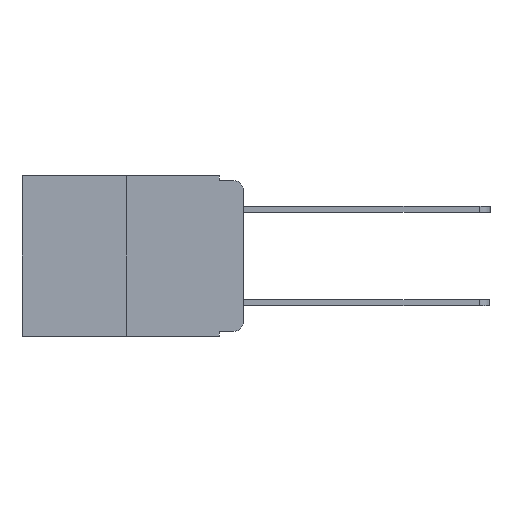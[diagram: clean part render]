
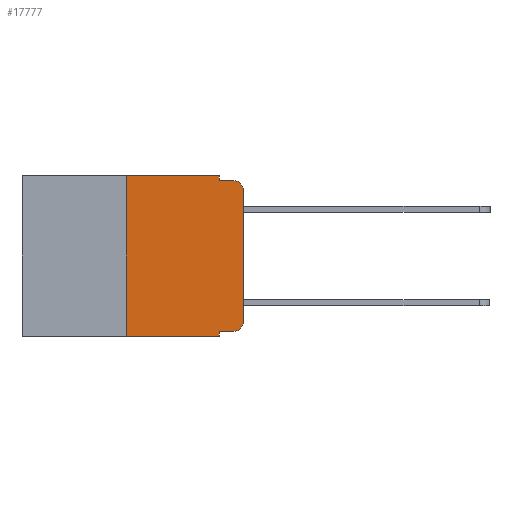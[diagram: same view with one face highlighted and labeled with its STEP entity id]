
A CAD part, left-side view. The second image highlights one B-rep face of the part: STEP entity #17777.
In plain terms, the highlighted planar face has unit normal (-1, 0, 0).
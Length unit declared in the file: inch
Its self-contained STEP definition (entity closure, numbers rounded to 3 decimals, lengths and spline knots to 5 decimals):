
#279 = VECTOR ( 'NONE', #8075, 39.37008 ) ;
#639 = ORIENTED_EDGE ( 'NONE', *, *, #17672, .T. ) ;
#662 = VERTEX_POINT ( 'NONE', #15641 ) ;
#718 = DIRECTION ( 'NONE',  ( 0., -1., 0. ) ) ;
#961 = AXIS2_PLACEMENT_3D ( 'NONE', #13818, #5654, #15170 ) ;
#1126 = AXIS2_PLACEMENT_3D ( 'NONE', #16324, #8238, #17665 ) ;
#1350 = ORIENTED_EDGE ( 'NONE', *, *, #10837, .F. ) ;
#1382 = PLANE ( 'NONE',  #961 ) ;
#1515 = CARTESIAN_POINT ( 'NONE',  ( 0., 0., -0.313 ) ) ;
#1614 = FACE_OUTER_BOUND ( 'NONE', #2027, .T. ) ;
#1800 = ORIENTED_EDGE ( 'NONE', *, *, #10014, .T. ) ;
#2027 = EDGE_LOOP ( 'NONE', ( #1800, #17594, #4031, #15746, #5764, #1350, #6407, #3618, #639, #6210 ) ) ;
#2047 = CARTESIAN_POINT ( 'NONE',  ( 0., 0.051, -0.343 ) ) ;
#2049 = DIRECTION ( 'NONE',  ( -1., 0., 0. ) ) ;
#2237 = VECTOR ( 'NONE', #15881, 39.37008 ) ;
#2392 = DIRECTION ( 'NONE',  ( 0., -1., 0. ) ) ;
#2447 = CIRCLE ( 'NONE', #1126, 0.02 ) ;
#2572 = VERTEX_POINT ( 'NONE', #16984 ) ;
#2578 = VECTOR ( 'NONE', #5127, 39.37008 ) ;
#2597 = CARTESIAN_POINT ( 'NONE',  ( 0., 0.051, -0.333 ) ) ;
#2837 = VERTEX_POINT ( 'NONE', #9090 ) ;
#3618 = ORIENTED_EDGE ( 'NONE', *, *, #13225, .F. ) ;
#3702 = CARTESIAN_POINT ( 'NONE',  ( 0., 0.051, -0.01 ) ) ;
#3815 = CARTESIAN_POINT ( 'NONE',  ( 0., 0., -0.03 ) ) ;
#3895 = VERTEX_POINT ( 'NONE', #6278 ) ;
#4012 = DIRECTION ( 'NONE',  ( 0., -1., 0. ) ) ;
#4031 = ORIENTED_EDGE ( 'NONE', *, *, #7508, .F. ) ;
#4441 = CARTESIAN_POINT ( 'NONE',  ( 0., 0.051, 0. ) ) ;
#4512 = CARTESIAN_POINT ( 'NONE',  ( 0., 0.25, 0. ) ) ;
#4763 = VECTOR ( 'NONE', #15292, 39.37008 ) ;
#5018 = CARTESIAN_POINT ( 'NONE',  ( 0., 0.051, 0. ) ) ;
#5127 = DIRECTION ( 'NONE',  ( 0., -1., 0. ) ) ;
#5654 = DIRECTION ( 'NONE',  ( 1., 0., 0. ) ) ;
#5764 = ORIENTED_EDGE ( 'NONE', *, *, #13348, .F. ) ;
#5766 = LINE ( 'NONE', #4441, #8536 ) ;
#6210 = ORIENTED_EDGE ( 'NONE', *, *, #8307, .T. ) ;
#6259 = CIRCLE ( 'NONE', #12583, 0.02 ) ;
#6276 = LINE ( 'NONE', #13308, #2578 ) ;
#6278 = CARTESIAN_POINT ( 'NONE',  ( 0., 0.051, 0. ) ) ;
#6372 = LINE ( 'NONE', #5018, #2237 ) ;
#6392 = VECTOR ( 'NONE', #718, 39.37008 ) ;
#6407 = ORIENTED_EDGE ( 'NONE', *, *, #10538, .T. ) ;
#6731 = CARTESIAN_POINT ( 'NONE',  ( 0., 0., 0. ) ) ;
#7066 = VECTOR ( 'NONE', #4012, 39.37008 ) ;
#7508 = EDGE_CURVE ( 'NONE', #16400, #7605, #14688, .T. ) ;
#7605 = VERTEX_POINT ( 'NONE', #13563 ) ;
#7802 = LINE ( 'NONE', #6731, #279 ) ;
#7900 = CARTESIAN_POINT ( 'NONE',  ( 0., 0.051, -0.01 ) ) ;
#8075 = DIRECTION ( 'NONE',  ( 0., 0., 1. ) ) ;
#8078 = EDGE_CURVE ( 'NONE', #3895, #16400, #6372, .T. ) ;
#8238 = DIRECTION ( 'NONE',  ( -1., 0., 0. ) ) ;
#8307 = EDGE_CURVE ( 'NONE', #2572, #13183, #2447, .T. ) ;
#8391 = LINE ( 'NONE', #13955, #4763 ) ;
#8536 = VECTOR ( 'NONE', #15351, 39.37008 ) ;
#9090 = CARTESIAN_POINT ( 'NONE',  ( 0., 0.051, -0.333 ) ) ;
#9122 = CARTESIAN_POINT ( 'NONE',  ( 0., 0.473, 0. ) ) ;
#10014 = EDGE_CURVE ( 'NONE', #13183, #12296, #7802, .T. ) ;
#10041 = LINE ( 'NONE', #9122, #6392 ) ;
#10344 = CARTESIAN_POINT ( 'NONE',  ( 0., 0.02, -0.03 ) ) ;
#10538 = EDGE_CURVE ( 'NONE', #662, #12791, #6276, .T. ) ;
#10837 = EDGE_CURVE ( 'NONE', #662, #10880, #8391, .T. ) ;
#10880 = VERTEX_POINT ( 'NONE', #4512 ) ;
#11088 = VECTOR ( 'NONE', #2392, 39.37008 ) ;
#11169 = LINE ( 'NONE', #2597, #7066 ) ;
#11727 = DIRECTION ( 'NONE',  ( 0., 0., -1. ) ) ;
#12296 = VERTEX_POINT ( 'NONE', #3815 ) ;
#12583 = AXIS2_PLACEMENT_3D ( 'NONE', #10344, #2049, #11727 ) ;
#12791 = VERTEX_POINT ( 'NONE', #2047 ) ;
#13183 = VERTEX_POINT ( 'NONE', #1515 ) ;
#13225 = EDGE_CURVE ( 'NONE', #2837, #12791, #5766, .T. ) ;
#13308 = CARTESIAN_POINT ( 'NONE',  ( 0., 0.473, -0.343 ) ) ;
#13348 = EDGE_CURVE ( 'NONE', #10880, #3895, #10041, .T. ) ;
#13563 = CARTESIAN_POINT ( 'NONE',  ( 0., 0.02, -0.01 ) ) ;
#13818 = CARTESIAN_POINT ( 'NONE',  ( 0., 0.473, 0. ) ) ;
#13955 = CARTESIAN_POINT ( 'NONE',  ( 0., 0.25, 0. ) ) ;
#14688 = LINE ( 'NONE', #7900, #11088 ) ;
#15170 = DIRECTION ( 'NONE',  ( 0., 0., -1. ) ) ;
#15292 = DIRECTION ( 'NONE',  ( 0., 0., 1. ) ) ;
#15351 = DIRECTION ( 'NONE',  ( 0., 0., -1. ) ) ;
#15641 = CARTESIAN_POINT ( 'NONE',  ( 0., 0.25, -0.343 ) ) ;
#15746 = ORIENTED_EDGE ( 'NONE', *, *, #8078, .F. ) ;
#15881 = DIRECTION ( 'NONE',  ( 0., 0., -1. ) ) ;
#16324 = CARTESIAN_POINT ( 'NONE',  ( 0., 0.02, -0.313 ) ) ;
#16400 = VERTEX_POINT ( 'NONE', #3702 ) ;
#16898 = EDGE_CURVE ( 'NONE', #12296, #7605, #6259, .T. ) ;
#16984 = CARTESIAN_POINT ( 'NONE',  ( 0., 0.02, -0.333 ) ) ;
#17594 = ORIENTED_EDGE ( 'NONE', *, *, #16898, .T. ) ;
#17665 = DIRECTION ( 'NONE',  ( 0., 0., -1. ) ) ;
#17672 = EDGE_CURVE ( 'NONE', #2837, #2572, #11169, .T. ) ;
#17777 = ADVANCED_FACE ( 'NONE', ( #1614 ), #1382, .F. ) ;
